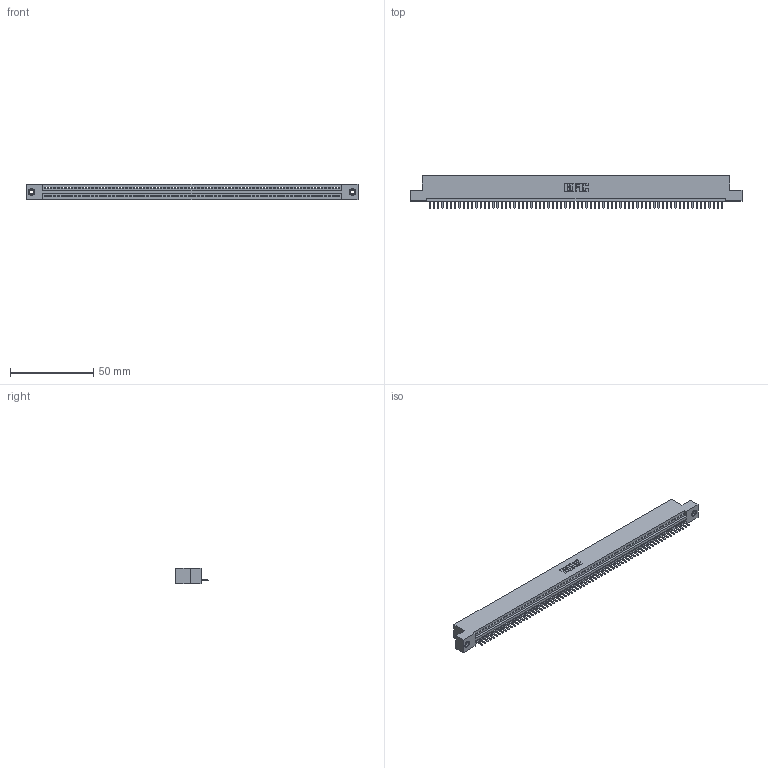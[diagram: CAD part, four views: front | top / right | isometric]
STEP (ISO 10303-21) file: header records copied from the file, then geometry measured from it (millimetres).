
FILE_DESCRIPTION (( 'STEP AP203' ), '1' );
FILE_NAME ('395-070-520-108.STEP', '2019-10-25T22:54:15', ( '' ), ( '' ), 'SwSTEP 2.0', 'SolidWorks 2016', '' );
FILE_SCHEMA (( 'CONFIG_CONTROL_DESIGN' ));
Length unit declared in the file: inch
Products named in the file (4): 345-292-001_345-293-120; 345 Part_Flush Mounting Lugs - 0.156 Dia-TI; 345-250-001_345-250-003-102; 395-070-520-108
Assembly tree (73 placements, depth 2):
  395-070-520-108
    345 Part_Flush Mounting Lugs - 0.156 Dia-TI
    345-292-001_345-293-120  x70
    345-250-001_345-250-003-102  x2
Bounding box: 199.01 x 19.68 x 9.4 mm (x, y, z)
Volume: 18923.6 mm3; surface area: 24888.7 mm2
Topology: 73 solids, 73 shells, 4526 faces, 13357 edges, 8710 vertices
Faces by surface type: plane 3052, cylinder 1458, cone 12, torus 4
Entity records: 50214 total; most frequent: CARTESIAN_POINT 8689, ORIENTED_EDGE 8674, DIRECTION 7563, EDGE_CURVE 4337, LINE 3901, VECTOR 3901, VERTEX_POINT 2884, AXIS2_PLACEMENT_3D 1831
